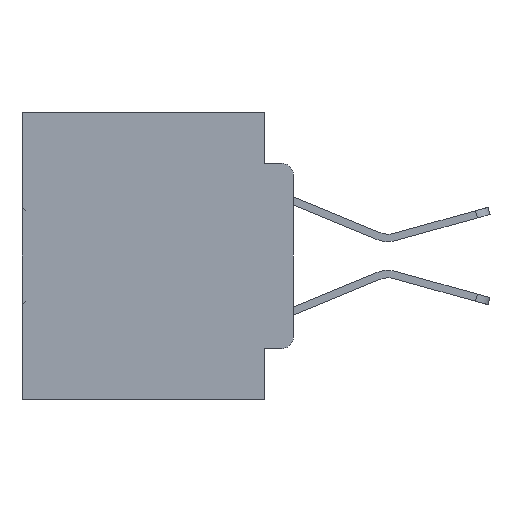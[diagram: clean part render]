
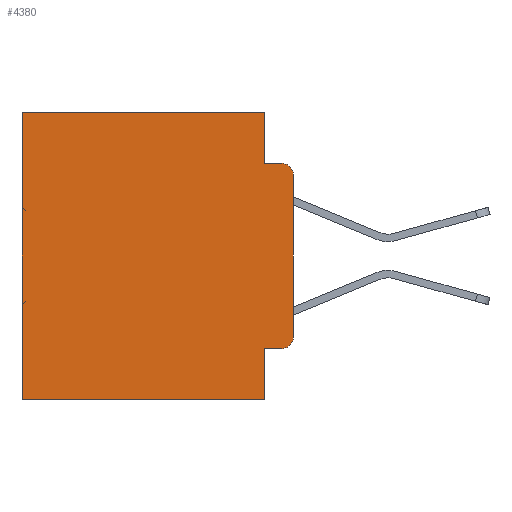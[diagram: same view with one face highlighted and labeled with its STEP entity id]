
A CAD part, left-side view. The second image highlights one B-rep face of the part: STEP entity #4380.
In plain terms, the highlighted planar face has unit normal (-1, 0, 0).
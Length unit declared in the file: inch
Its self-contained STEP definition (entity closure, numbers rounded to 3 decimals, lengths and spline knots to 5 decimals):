
#14 = VERTEX_POINT ( 'NONE', #15265 ) ;
#35 = VECTOR ( 'NONE', #10396, 39.37008 ) ;
#340 = CARTESIAN_POINT ( 'NONE',  ( 0.298, 0.051, 0. ) ) ;
#737 = DIRECTION ( 'NONE',  ( 0., 1., 0. ) ) ;
#1541 = CIRCLE ( 'NONE', #17926, 0.02 ) ;
#1653 = VERTEX_POINT ( 'NONE', #2269 ) ;
#1683 = LINE ( 'NONE', #28524, #25219 ) ;
#1847 = DIRECTION ( 'NONE',  ( -1., 0., 0. ) ) ;
#1896 = VERTEX_POINT ( 'NONE', #3332 ) ;
#2019 = DIRECTION ( 'NONE',  ( 0., 0., -1. ) ) ;
#2269 = CARTESIAN_POINT ( 'NONE',  ( 0.298, 0.473, 0. ) ) ;
#2424 = CARTESIAN_POINT ( 'NONE',  ( 0.298, 0.051, -0.0885 ) ) ;
#3332 = CARTESIAN_POINT ( 'NONE',  ( 0.298, 0., -0.1085 ) ) ;
#3544 = VERTEX_POINT ( 'NONE', #2424 ) ;
#4380 = ADVANCED_FACE ( 'NONE', ( #13611 ), #23667, .F. ) ;
#4757 = AXIS2_PLACEMENT_3D ( 'NONE', #18737, #29647, #26850 ) ;
#5007 = CARTESIAN_POINT ( 'NONE',  ( 0.298, 0.02, -0.3915 ) ) ;
#5185 = VERTEX_POINT ( 'NONE', #21863 ) ;
#5619 = VECTOR ( 'NONE', #25073, 39.37008 ) ;
#6012 = VERTEX_POINT ( 'NONE', #29204 ) ;
#7047 = DIRECTION ( 'NONE',  ( 0., 0., -1. ) ) ;
#7147 = EDGE_CURVE ( 'NONE', #23299, #3544, #7185, .T. ) ;
#7185 = LINE ( 'NONE', #12329, #29530 ) ;
#8456 = AXIS2_PLACEMENT_3D ( 'NONE', #5007, #1847, #2019 ) ;
#8833 = LINE ( 'NONE', #25593, #5619 ) ;
#10396 = DIRECTION ( 'NONE',  ( 0., 0., -1. ) ) ;
#11177 = ORIENTED_EDGE ( 'NONE', *, *, #7147, .F. ) ;
#12050 = VECTOR ( 'NONE', #7047, 39.37008 ) ;
#12329 = CARTESIAN_POINT ( 'NONE',  ( 0.298, 0.051, 0. ) ) ;
#13131 = CARTESIAN_POINT ( 'NONE',  ( 0.298, 0.051, -0.0885 ) ) ;
#13492 = LINE ( 'NONE', #13131, #30894 ) ;
#13611 = FACE_OUTER_BOUND ( 'NONE', #31153, .T. ) ;
#13955 = ORIENTED_EDGE ( 'NONE', *, *, #24469, .F. ) ;
#14196 = LINE ( 'NONE', #14370, #25220 ) ;
#14370 = CARTESIAN_POINT ( 'NONE',  ( 0.298, 0., -0.5 ) ) ;
#14695 = CARTESIAN_POINT ( 'NONE',  ( 0.298, 0., 0. ) ) ;
#15265 = CARTESIAN_POINT ( 'NONE',  ( 0.298, 0.051, -0.4115 ) ) ;
#15625 = CARTESIAN_POINT ( 'NONE',  ( 0.298, 0.051, -0.5 ) ) ;
#15793 = ORIENTED_EDGE ( 'NONE', *, *, #28842, .F. ) ;
#15956 = ORIENTED_EDGE ( 'NONE', *, *, #21063, .F. ) ;
#16499 = ORIENTED_EDGE ( 'NONE', *, *, #20589, .T. ) ;
#16903 = EDGE_CURVE ( 'NONE', #14, #6012, #1683, .T. ) ;
#16918 = CARTESIAN_POINT ( 'NONE',  ( 0.298, 0.051, 0. ) ) ;
#16963 = LINE ( 'NONE', #27719, #29977 ) ;
#17505 = EDGE_CURVE ( 'NONE', #1896, #5185, #1541, .T. ) ;
#17926 = AXIS2_PLACEMENT_3D ( 'NONE', #26380, #20733, #34483 ) ;
#18545 = LINE ( 'NONE', #340, #35 ) ;
#18549 = ORIENTED_EDGE ( 'NONE', *, *, #19097, .T. ) ;
#18737 = CARTESIAN_POINT ( 'NONE',  ( 0.298, 0., 0. ) ) ;
#19097 = EDGE_CURVE ( 'NONE', #1653, #19524, #8833, .T. ) ;
#19203 = VERTEX_POINT ( 'NONE', #23444 ) ;
#19524 = VERTEX_POINT ( 'NONE', #19761 ) ;
#19761 = CARTESIAN_POINT ( 'NONE',  ( 0.298, 0.473, -0.5 ) ) ;
#20589 = EDGE_CURVE ( 'NONE', #6012, #19203, #32735, .T. ) ;
#20733 = DIRECTION ( 'NONE',  ( -1., 0., 0. ) ) ;
#21063 = EDGE_CURVE ( 'NONE', #14, #34031, #18545, .T. ) ;
#21863 = CARTESIAN_POINT ( 'NONE',  ( 0.298, 0.02, -0.0885 ) ) ;
#22802 = EDGE_CURVE ( 'NONE', #23299, #1653, #16963, .T. ) ;
#23299 = VERTEX_POINT ( 'NONE', #16918 ) ;
#23444 = CARTESIAN_POINT ( 'NONE',  ( 0.298, 0., -0.3915 ) ) ;
#23667 = PLANE ( 'NONE',  #4757 ) ;
#24469 = EDGE_CURVE ( 'NONE', #1896, #19203, #33905, .T. ) ;
#25073 = DIRECTION ( 'NONE',  ( 0., 0., -1. ) ) ;
#25219 = VECTOR ( 'NONE', #25373, 39.37008 ) ;
#25220 = VECTOR ( 'NONE', #737, 39.37008 ) ;
#25373 = DIRECTION ( 'NONE',  ( 0., -1., 0. ) ) ;
#25593 = CARTESIAN_POINT ( 'NONE',  ( 0.298, 0.473, 0. ) ) ;
#26380 = CARTESIAN_POINT ( 'NONE',  ( 0.298, 0.02, -0.1085 ) ) ;
#26551 = DIRECTION ( 'NONE',  ( 0., -1., 0. ) ) ;
#26850 = DIRECTION ( 'NONE',  ( 0., 0., -1. ) ) ;
#27719 = CARTESIAN_POINT ( 'NONE',  ( 0.298, 0., 0. ) ) ;
#27915 = ORIENTED_EDGE ( 'NONE', *, *, #16903, .T. ) ;
#28047 = DIRECTION ( 'NONE',  ( 0., 0., -1. ) ) ;
#28524 = CARTESIAN_POINT ( 'NONE',  ( 0.298, 0.051, -0.4115 ) ) ;
#28571 = DIRECTION ( 'NONE',  ( 0., 1., 0. ) ) ;
#28842 = EDGE_CURVE ( 'NONE', #34031, #19524, #14196, .T. ) ;
#29204 = CARTESIAN_POINT ( 'NONE',  ( 0.298, 0.02, -0.4115 ) ) ;
#29530 = VECTOR ( 'NONE', #28047, 39.37008 ) ;
#29647 = DIRECTION ( 'NONE',  ( 1., 0., 0. ) ) ;
#29977 = VECTOR ( 'NONE', #28571, 39.37008 ) ;
#30001 = EDGE_CURVE ( 'NONE', #3544, #5185, #13492, .T. ) ;
#30499 = ORIENTED_EDGE ( 'NONE', *, *, #22802, .T. ) ;
#30894 = VECTOR ( 'NONE', #26551, 39.37008 ) ;
#31153 = EDGE_LOOP ( 'NONE', ( #13955, #31940, #34822, #11177, #30499, #18549, #15793, #15956, #27915, #16499 ) ) ;
#31940 = ORIENTED_EDGE ( 'NONE', *, *, #17505, .T. ) ;
#32735 = CIRCLE ( 'NONE', #8456, 0.02 ) ;
#33905 = LINE ( 'NONE', #14695, #12050 ) ;
#34031 = VERTEX_POINT ( 'NONE', #15625 ) ;
#34483 = DIRECTION ( 'NONE',  ( 0., 0., -1. ) ) ;
#34822 = ORIENTED_EDGE ( 'NONE', *, *, #30001, .F. ) ;
